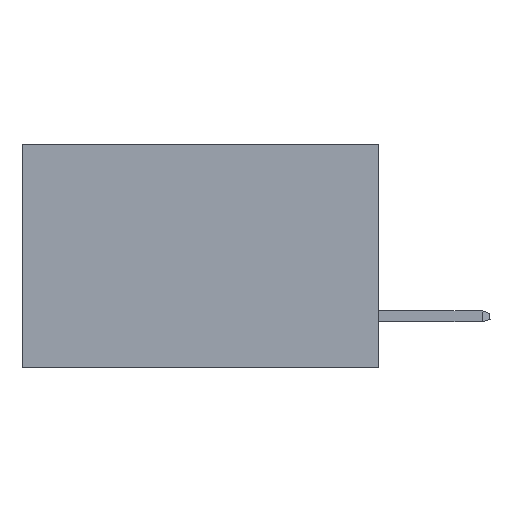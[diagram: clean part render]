
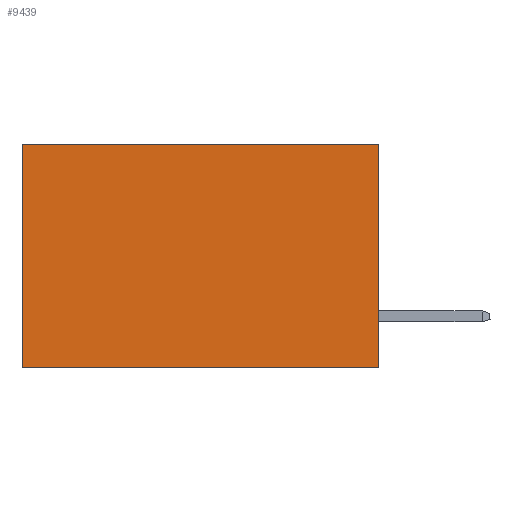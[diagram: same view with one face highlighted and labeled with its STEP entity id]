
A CAD part, left-side view. The second image highlights one B-rep face of the part: STEP entity #9439.
In plain terms, the highlighted planar face has unit normal (-1, 0, 0).
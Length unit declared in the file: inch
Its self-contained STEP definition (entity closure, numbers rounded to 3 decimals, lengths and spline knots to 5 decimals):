
#310 = ORIENTED_EDGE ( 'NONE', *, *, #4211, .F. ) ;
#360 = CARTESIAN_POINT ( 'NONE',  ( 0.277, 0., -0.37 ) ) ;
#389 = EDGE_CURVE ( 'NONE', #6191, #6170, #9164, .T. ) ;
#1300 = LINE ( 'NONE', #8073, #10356 ) ;
#1470 = ORIENTED_EDGE ( 'NONE', *, *, #3480, .F. ) ;
#1527 = FACE_OUTER_BOUND ( 'NONE', #5705, .T. ) ;
#1643 = VECTOR ( 'NONE', #9994, 39.37008 ) ;
#3479 = LINE ( 'NONE', #3911, #1643 ) ;
#3480 = EDGE_CURVE ( 'NONE', #7346, #6170, #3479, .T. ) ;
#3717 = DIRECTION ( 'NONE',  ( 0., 0., -1. ) ) ;
#3911 = CARTESIAN_POINT ( 'NONE',  ( 0.277, 0., -0.37 ) ) ;
#4196 = VECTOR ( 'NONE', #3717, 39.37008 ) ;
#4197 = PLANE ( 'NONE',  #6233 ) ;
#4211 = EDGE_CURVE ( 'NONE', #5059, #7346, #11189, .T. ) ;
#4442 = CARTESIAN_POINT ( 'NONE',  ( 0.277, 0., 0. ) ) ;
#5038 = CARTESIAN_POINT ( 'NONE',  ( 0.277, 0., -0.37 ) ) ;
#5059 = VERTEX_POINT ( 'NONE', #4442 ) ;
#5074 = DIRECTION ( 'NONE',  ( 1., 0., 0. ) ) ;
#5705 = EDGE_LOOP ( 'NONE', ( #7591, #1470, #310, #9287 ) ) ;
#6170 = VERTEX_POINT ( 'NONE', #6254 ) ;
#6191 = VERTEX_POINT ( 'NONE', #7237 ) ;
#6233 = AXIS2_PLACEMENT_3D ( 'NONE', #5038, #5074, #11116 ) ;
#6254 = CARTESIAN_POINT ( 'NONE',  ( 0.277, 0.59, -0.37 ) ) ;
#6307 = CARTESIAN_POINT ( 'NONE',  ( 0.277, 0., -0.37 ) ) ;
#6827 = EDGE_CURVE ( 'NONE', #5059, #6191, #1300, .T. ) ;
#7237 = CARTESIAN_POINT ( 'NONE',  ( 0.277, 0.59, 0. ) ) ;
#7346 = VERTEX_POINT ( 'NONE', #6307 ) ;
#7591 = ORIENTED_EDGE ( 'NONE', *, *, #389, .T. ) ;
#8073 = CARTESIAN_POINT ( 'NONE',  ( 0.277, 0., 0. ) ) ;
#8407 = DIRECTION ( 'NONE',  ( 0., 0., -1. ) ) ;
#8882 = CARTESIAN_POINT ( 'NONE',  ( 0.277, 0.59, -0.37 ) ) ;
#9164 = LINE ( 'NONE', #8882, #4196 ) ;
#9287 = ORIENTED_EDGE ( 'NONE', *, *, #6827, .T. ) ;
#9439 = ADVANCED_FACE ( 'NONE', ( #1527 ), #4197, .F. ) ;
#9994 = DIRECTION ( 'NONE',  ( 0., 1., 0. ) ) ;
#10356 = VECTOR ( 'NONE', #10624, 39.37008 ) ;
#10624 = DIRECTION ( 'NONE',  ( 0., 1., 0. ) ) ;
#10920 = VECTOR ( 'NONE', #8407, 39.37008 ) ;
#11116 = DIRECTION ( 'NONE',  ( 0., 0., -1. ) ) ;
#11189 = LINE ( 'NONE', #360, #10920 ) ;
